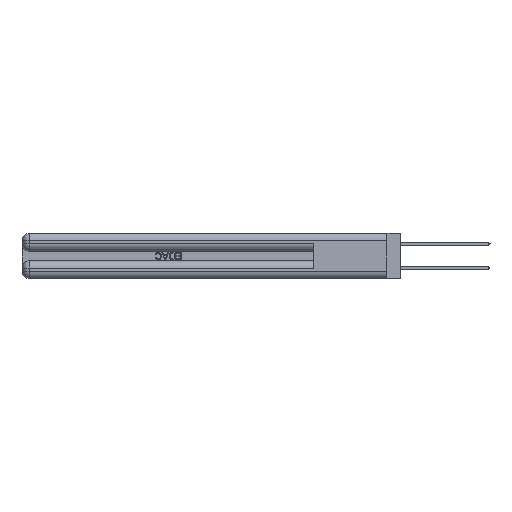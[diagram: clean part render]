
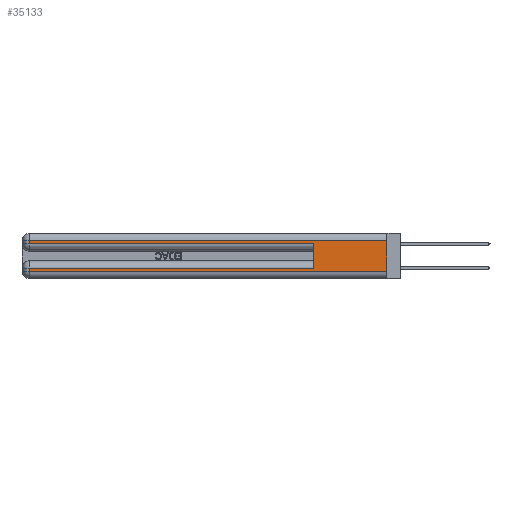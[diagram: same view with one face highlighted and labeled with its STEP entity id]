
A CAD part, left-side view. The second image highlights one B-rep face of the part: STEP entity #35133.
In plain terms, the highlighted planar face has unit normal (-1, 0, 0).
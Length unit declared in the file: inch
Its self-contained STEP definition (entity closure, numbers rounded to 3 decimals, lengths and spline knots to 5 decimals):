
#933 = ORIENTED_EDGE ( 'NONE', *, *, #9302, .T. ) ;
#1485 = EDGE_CURVE ( 'NONE', #15104, #10440, #44958, .T. ) ;
#1515 = ORIENTED_EDGE ( 'NONE', *, *, #25042, .T. ) ;
#1634 = VERTEX_POINT ( 'NONE', #15740 ) ;
#3016 = CARTESIAN_POINT ( 'NONE',  ( 0., 0., 0.085 ) ) ;
#4111 = CARTESIAN_POINT ( 'NONE',  ( 0., 2.94, 0.37 ) ) ;
#4233 = CARTESIAN_POINT ( 'NONE',  ( 0., 0., 0.06 ) ) ;
#5308 = CARTESIAN_POINT ( 'NONE',  ( 0., 0., 0.37 ) ) ;
#7139 = CARTESIAN_POINT ( 'NONE',  ( 0., 2.94, 0.085 ) ) ;
#8770 = CARTESIAN_POINT ( 'NONE',  ( 0., 0., 0.37 ) ) ;
#9197 = CARTESIAN_POINT ( 'NONE',  ( 0., 0., 0.31 ) ) ;
#9302 = EDGE_CURVE ( 'NONE', #1634, #41663, #30040, .T. ) ;
#10440 = VERTEX_POINT ( 'NONE', #7139 ) ;
#11130 = VECTOR ( 'NONE', #13097, 39.37008 ) ;
#12169 = VECTOR ( 'NONE', #13430, 39.37008 ) ;
#12620 = DIRECTION ( 'NONE',  ( 0., 0., -1. ) ) ;
#13097 = DIRECTION ( 'NONE',  ( 0., 0., -1. ) ) ;
#13430 = DIRECTION ( 'NONE',  ( 0., 0., 1. ) ) ;
#13632 = VECTOR ( 'NONE', #35045, 39.37008 ) ;
#14599 = CARTESIAN_POINT ( 'NONE',  ( 0., 2.94, 0.31 ) ) ;
#15104 = VERTEX_POINT ( 'NONE', #20387 ) ;
#15740 = CARTESIAN_POINT ( 'NONE',  ( 0., 2.94, 0.06 ) ) ;
#16085 = AXIS2_PLACEMENT_3D ( 'NONE', #8770, #35716, #12620 ) ;
#16484 = LINE ( 'NONE', #25450, #46042 ) ;
#16525 = EDGE_LOOP ( 'NONE', ( #18497, #28799, #1515, #22153, #23382, #36025, #16700, #933 ) ) ;
#16700 = ORIENTED_EDGE ( 'NONE', *, *, #22896, .T. ) ;
#18497 = ORIENTED_EDGE ( 'NONE', *, *, #33290, .F. ) ;
#18873 = DIRECTION ( 'NONE',  ( 0., -1., 0. ) ) ;
#19706 = CARTESIAN_POINT ( 'NONE',  ( 0., 2.94, 0.285 ) ) ;
#19888 = LINE ( 'NONE', #46787, #48189 ) ;
#20387 = CARTESIAN_POINT ( 'NONE',  ( 0., 0.6, 0.085 ) ) ;
#21353 = LINE ( 'NONE', #5308, #11130 ) ;
#22153 = ORIENTED_EDGE ( 'NONE', *, *, #31462, .T. ) ;
#22440 = LINE ( 'NONE', #28832, #12169 ) ;
#22896 = EDGE_CURVE ( 'NONE', #10440, #1634, #23938, .T. ) ;
#23382 = ORIENTED_EDGE ( 'NONE', *, *, #35298, .F. ) ;
#23759 = DIRECTION ( 'NONE',  ( 0., -1., 0. ) ) ;
#23938 = LINE ( 'NONE', #4111, #13632 ) ;
#24543 = LINE ( 'NONE', #26314, #43808 ) ;
#25042 = EDGE_CURVE ( 'NONE', #33539, #33084, #16484, .T. ) ;
#25450 = CARTESIAN_POINT ( 'NONE',  ( 0., 2.94, 0.37 ) ) ;
#26242 = DIRECTION ( 'NONE',  ( 0., 1., 0. ) ) ;
#26314 = CARTESIAN_POINT ( 'NONE',  ( 0., 0., 0.31 ) ) ;
#28799 = ORIENTED_EDGE ( 'NONE', *, *, #40951, .T. ) ;
#28832 = CARTESIAN_POINT ( 'NONE',  ( 0., 0.6, 0.145 ) ) ;
#30040 = LINE ( 'NONE', #38099, #39048 ) ;
#30185 = DIRECTION ( 'NONE',  ( 0., 1., 0. ) ) ;
#31462 = EDGE_CURVE ( 'NONE', #33084, #46216, #19888, .T. ) ;
#33084 = VERTEX_POINT ( 'NONE', #19706 ) ;
#33290 = EDGE_CURVE ( 'NONE', #41884, #41663, #21353, .T. ) ;
#33539 = VERTEX_POINT ( 'NONE', #14599 ) ;
#35045 = DIRECTION ( 'NONE',  ( 0., 0., -1. ) ) ;
#35133 = ADVANCED_FACE ( 'NONE', ( #42354 ), #47146, .F. ) ;
#35298 = EDGE_CURVE ( 'NONE', #15104, #46216, #22440, .T. ) ;
#35716 = DIRECTION ( 'NONE',  ( 1., 0., 0. ) ) ;
#36025 = ORIENTED_EDGE ( 'NONE', *, *, #1485, .T. ) ;
#38099 = CARTESIAN_POINT ( 'NONE',  ( 0., 0., 0.06 ) ) ;
#39048 = VECTOR ( 'NONE', #18873, 39.37008 ) ;
#40774 = DIRECTION ( 'NONE',  ( 0., 0., -1. ) ) ;
#40951 = EDGE_CURVE ( 'NONE', #41884, #33539, #24543, .T. ) ;
#41663 = VERTEX_POINT ( 'NONE', #4233 ) ;
#41884 = VERTEX_POINT ( 'NONE', #9197 ) ;
#42354 = FACE_OUTER_BOUND ( 'NONE', #16525, .T. ) ;
#43808 = VECTOR ( 'NONE', #30185, 39.37008 ) ;
#44958 = LINE ( 'NONE', #3016, #47351 ) ;
#46042 = VECTOR ( 'NONE', #40774, 39.37008 ) ;
#46216 = VERTEX_POINT ( 'NONE', #48913 ) ;
#46787 = CARTESIAN_POINT ( 'NONE',  ( 0., 0., 0.285 ) ) ;
#47146 = PLANE ( 'NONE',  #16085 ) ;
#47351 = VECTOR ( 'NONE', #26242, 39.37008 ) ;
#48189 = VECTOR ( 'NONE', #23759, 39.37008 ) ;
#48913 = CARTESIAN_POINT ( 'NONE',  ( 0., 0.6, 0.285 ) ) ;
